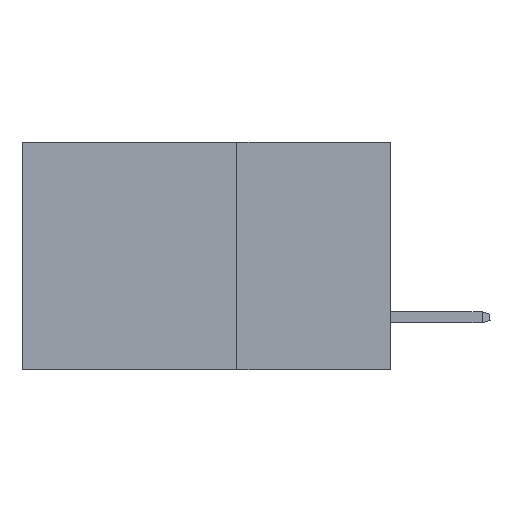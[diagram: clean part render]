
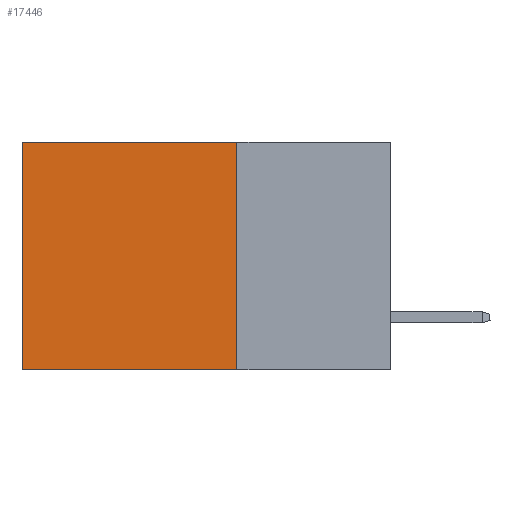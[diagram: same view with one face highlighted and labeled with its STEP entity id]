
A CAD part, left-side view. The second image highlights one B-rep face of the part: STEP entity #17446.
In plain terms, the highlighted planar face has unit normal (-1, 0, 0).
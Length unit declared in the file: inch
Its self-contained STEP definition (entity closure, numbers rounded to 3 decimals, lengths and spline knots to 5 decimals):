
#195 = ORIENTED_EDGE ( 'NONE', *, *, #18302, .T. ) ;
#781 = CARTESIAN_POINT ( 'NONE',  ( 0.2875, 0.25, -0.37 ) ) ;
#1118 = CARTESIAN_POINT ( 'NONE',  ( 0.2875, 0.25, -0.37 ) ) ;
#1281 = CARTESIAN_POINT ( 'NONE',  ( 0.2875, 0.6, -0.37 ) ) ;
#1628 = DIRECTION ( 'NONE',  ( 0., 0., -1. ) ) ;
#2306 = VERTEX_POINT ( 'NONE', #6941 ) ;
#2478 = DIRECTION ( 'NONE',  ( 0., 1., 0. ) ) ;
#3055 = LINE ( 'NONE', #18915, #14345 ) ;
#3241 = LINE ( 'NONE', #11615, #10203 ) ;
#3403 = VERTEX_POINT ( 'NONE', #17817 ) ;
#3580 = FACE_OUTER_BOUND ( 'NONE', #15249, .T. ) ;
#4830 = DIRECTION ( 'NONE',  ( 0., 0., -1. ) ) ;
#5739 = DIRECTION ( 'NONE',  ( 0., 0., -1. ) ) ;
#6801 = VERTEX_POINT ( 'NONE', #1281 ) ;
#6941 = CARTESIAN_POINT ( 'NONE',  ( 0.2875, 0.25, 0. ) ) ;
#7810 = PLANE ( 'NONE',  #13028 ) ;
#8141 = ORIENTED_EDGE ( 'NONE', *, *, #13914, .T. ) ;
#8674 = ORIENTED_EDGE ( 'NONE', *, *, #19649, .F. ) ;
#9143 = CARTESIAN_POINT ( 'NONE',  ( 0.2875, 0.25, 0. ) ) ;
#10203 = VECTOR ( 'NONE', #5739, 39.37008 ) ;
#10815 = CARTESIAN_POINT ( 'NONE',  ( 0.2875, 0.25, 0. ) ) ;
#11615 = CARTESIAN_POINT ( 'NONE',  ( 0.2875, 0.6, 0. ) ) ;
#11851 = EDGE_CURVE ( 'NONE', #2306, #18508, #16925, .T. ) ;
#13028 = AXIS2_PLACEMENT_3D ( 'NONE', #10815, #18546, #4830 ) ;
#13746 = ORIENTED_EDGE ( 'NONE', *, *, #11851, .F. ) ;
#13914 = EDGE_CURVE ( 'NONE', #3403, #6801, #3241, .T. ) ;
#14345 = VECTOR ( 'NONE', #15808, 39.37008 ) ;
#15249 = EDGE_LOOP ( 'NONE', ( #8141, #8674, #13746, #195 ) ) ;
#15808 = DIRECTION ( 'NONE',  ( 0., 1., 0. ) ) ;
#16925 = LINE ( 'NONE', #9143, #17395 ) ;
#17395 = VECTOR ( 'NONE', #1628, 39.37008 ) ;
#17446 = ADVANCED_FACE ( 'NONE', ( #3580 ), #7810, .F. ) ;
#17817 = CARTESIAN_POINT ( 'NONE',  ( 0.2875, 0.6, 0. ) ) ;
#18108 = LINE ( 'NONE', #781, #18596 ) ;
#18302 = EDGE_CURVE ( 'NONE', #2306, #3403, #3055, .T. ) ;
#18508 = VERTEX_POINT ( 'NONE', #1118 ) ;
#18546 = DIRECTION ( 'NONE',  ( 1., 0., 0. ) ) ;
#18596 = VECTOR ( 'NONE', #2478, 39.37008 ) ;
#18915 = CARTESIAN_POINT ( 'NONE',  ( 0.2875, 0.25, 0. ) ) ;
#19649 = EDGE_CURVE ( 'NONE', #18508, #6801, #18108, .T. ) ;
